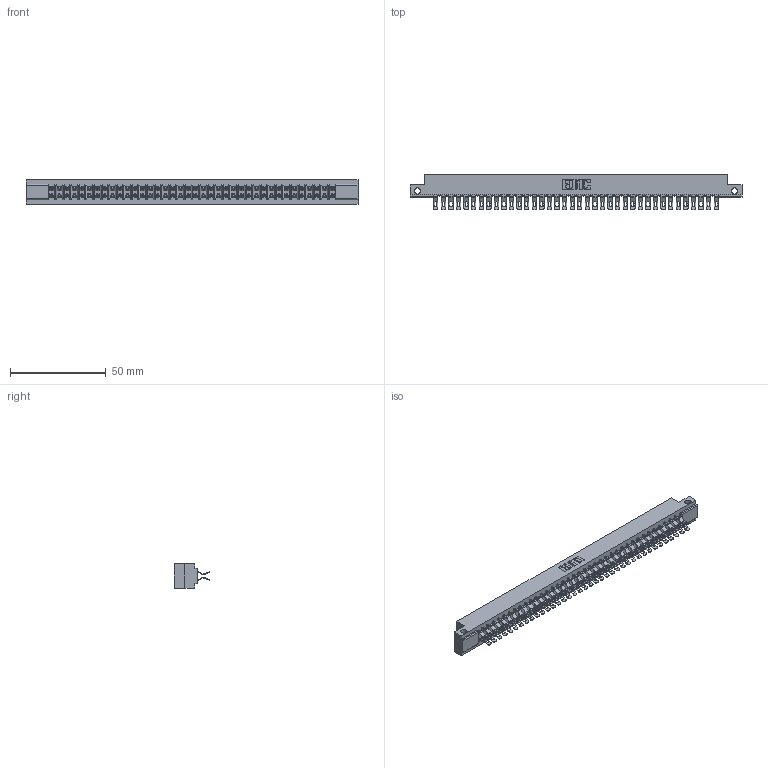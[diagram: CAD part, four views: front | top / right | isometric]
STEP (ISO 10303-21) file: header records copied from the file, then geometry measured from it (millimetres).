
FILE_DESCRIPTION (( 'STEP AP203' ), '1' );
FILE_NAME ('357-076-455-212.STEP', '2020-10-04T15:19:47', ( '' ), ( '' ), 'SwSTEP 2.0', 'SolidWorks 2020', '' );
FILE_SCHEMA (( 'CONFIG_CONTROL_DESIGN' ));
Length unit declared in the file: inch
Products named in the file (3): 307-290-001_555; 357-076-455-212; 307 Part_.128 Dia Side Mounting Holes
Assembly tree (77 placements, depth 2):
  357-076-455-212
    307 Part_.128 Dia Side Mounting Holes
    307-290-001_555  x76
Bounding box: 173.58 x 18.75 x 12.7 mm (x, y, z)
Volume: 18514.5 mm3; surface area: 23815.1 mm2
Topology: 77 solids, 77 shells, 4793 faces, 14079 edges, 9178 vertices
Faces by surface type: plane 2654, cylinder 2061, sphere 78
Entity records: 34825 total; most frequent: CARTESIAN_POINT 5702, ORIENTED_EDGE 5652, DIRECTION 5594, EDGE_CURVE 2826, VECTOR 2154, LINE 2154, VERTEX_POINT 1828, AXIS2_PLACEMENT_3D 1720
